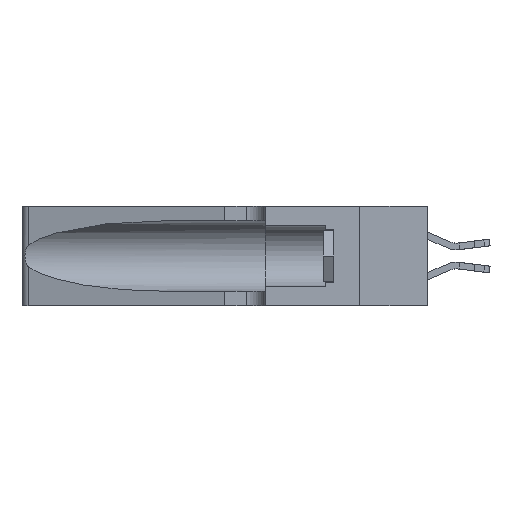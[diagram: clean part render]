
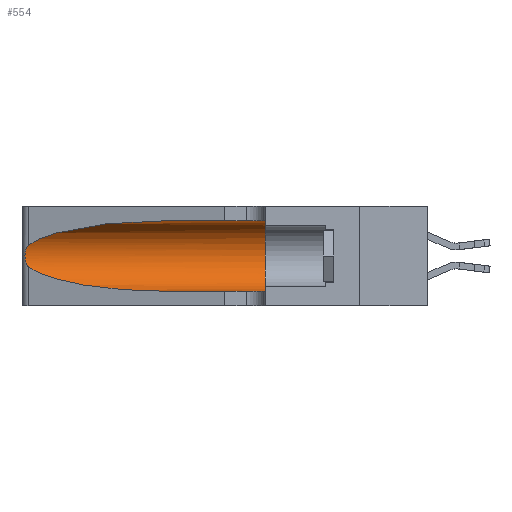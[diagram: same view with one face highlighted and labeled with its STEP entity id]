
A CAD part, left-side view. The second image highlights one B-rep face of the part: STEP entity #554.
In plain terms, the highlighted cylindrical face has radius 3.308 mm (diameter 6.617 mm), a partial arc.
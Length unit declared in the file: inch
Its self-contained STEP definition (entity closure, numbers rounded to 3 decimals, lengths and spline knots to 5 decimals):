
#235 = EDGE_LOOP ( 'NONE', ( #2622, #8775, #7417, #21664, #17510, #15327 ) ) ;
#342 = CARTESIAN_POINT ( 'NONE',  ( 0.25856, 1.23593, 0.16098 ) ) ;
#429 = CARTESIAN_POINT ( 'NONE',  ( 0.25487, 1.22718, 0.22369 ) ) ;
#525 = B_SPLINE_CURVE_WITH_KNOTS ( 'NONE', 3,
 ( #1756, #5209, #17364, #6971, #19101, #1903, #7247, #3805, #8969, #342, #2127, #16356, #9271, #3881 ),
 .UNSPECIFIED., .F., .F.,
 ( 4, 2, 2, 2, 2, 2, 4 ),
 ( 0., 0.00027, 0.00053, 0.00107, 0.0016, 0.00187, 0.00214 ),
 .UNSPECIFIED. ) ;
#554 = ADVANCED_FACE ( 'NONE', ( #5903 ), #7026, .F. ) ;
#969 = AXIS2_PLACEMENT_3D ( 'NONE', #9928, #2875, #3022 ) ;
#993 = VECTOR ( 'NONE', #12629, 39.37008 ) ;
#1394 = EDGE_CURVE ( 'NONE', #18174, #13818, #16700, .T. ) ;
#1395 = VERTEX_POINT ( 'NONE', #17748 ) ;
#1473 = CARTESIAN_POINT ( 'NONE',  ( 0.1305, 0.35, 0.05475 ) ) ;
#1756 = CARTESIAN_POINT ( 'NONE',  ( 0.25487, 1.22718, 0.22369 ) ) ;
#1782 = CARTESIAN_POINT ( 'NONE',  ( 0.25487, 1.22718, 0.14631 ) ) ;
#1903 = CARTESIAN_POINT ( 'NONE',  ( 0.26018, 1.23835, 0.19895 ) ) ;
#2127 = CARTESIAN_POINT ( 'NONE',  ( 0.25789, 1.23486, 0.15765 ) ) ;
#2622 = ORIENTED_EDGE ( 'NONE', *, *, #1394, .T. ) ;
#2875 = DIRECTION ( 'NONE',  ( 0., 1., 0. ) ) ;
#2895 = VERTEX_POINT ( 'NONE', #19126 ) ;
#2915 =( BOUNDED_CURVE ( )  B_SPLINE_CURVE ( 3, ( #1782, #10401, #10469, #22448 ),
 .UNSPECIFIED., .F., .F. ) 
 B_SPLINE_CURVE_WITH_KNOTS ( ( 4, 4 ),
 ( 3.44316, 4.71239 ),
 .UNSPECIFIED. ) 
 CURVE ( )  GEOMETRIC_REPRESENTATION_ITEM ( )  RATIONAL_B_SPLINE_CURVE ( ( 1., 0.87, 0.87, 1. ) ) 
 REPRESENTATION_ITEM ( '' )  );
#3022 = DIRECTION ( 'NONE',  ( 0., 0., 1. ) ) ;
#3223 = DIRECTION ( 'NONE',  ( 0., 0., -1. ) ) ;
#3502 = DIRECTION ( 'NONE',  ( 0., -1., 0. ) ) ;
#3805 = CARTESIAN_POINT ( 'NONE',  ( 0.26075, 1.23896, 0.178 ) ) ;
#3881 = CARTESIAN_POINT ( 'NONE',  ( 0.25487, 1.22718, 0.14631 ) ) ;
#3979 = CARTESIAN_POINT ( 'NONE',  ( 0.2373, 1.15595, 0.28018 ) ) ;
#5209 = CARTESIAN_POINT ( 'NONE',  ( 0.25555, 1.22994, 0.2215 ) ) ;
#5401 = LINE ( 'NONE', #12109, #21978 ) ;
#5612 = LINE ( 'NONE', #14020, #993 ) ;
#5903 = FACE_OUTER_BOUND ( 'NONE', #235, .T. ) ;
#6422 = CARTESIAN_POINT ( 'NONE',  ( 0.25487, 1.22718, 0.22369 ) ) ;
#6939 = CARTESIAN_POINT ( 'NONE',  ( 0.1305, 1.61858, 0.185 ) ) ;
#6971 = CARTESIAN_POINT ( 'NONE',  ( 0.25787, 1.23484, 0.2124 ) ) ;
#7026 = CYLINDRICAL_SURFACE ( 'NONE', #12128, 0.13025 ) ;
#7247 = CARTESIAN_POINT ( 'NONE',  ( 0.26075, 1.23896, 0.19203 ) ) ;
#7417 = ORIENTED_EDGE ( 'NONE', *, *, #16127, .T. ) ;
#8775 = ORIENTED_EDGE ( 'NONE', *, *, #13025, .T. ) ;
#8969 = CARTESIAN_POINT ( 'NONE',  ( 0.26017, 1.23833, 0.17102 ) ) ;
#9271 = CARTESIAN_POINT ( 'NONE',  ( 0.25555, 1.22993, 0.14849 ) ) ;
#9588 = VERTEX_POINT ( 'NONE', #15658 ) ;
#9928 = CARTESIAN_POINT ( 'NONE',  ( 0.1305, 0.35, 0.185 ) ) ;
#10401 = CARTESIAN_POINT ( 'NONE',  ( 0.2373, 1.15595, 0.08982 ) ) ;
#10469 = CARTESIAN_POINT ( 'NONE',  ( 0.18966, 0.96281, 0.05475 ) ) ;
#10640 = CIRCLE ( 'NONE', #969, 0.13025 ) ;
#10826 = CARTESIAN_POINT ( 'NONE',  ( 0.18966, 0.96281, 0.31525 ) ) ;
#12028 = VERTEX_POINT ( 'NONE', #1473 ) ;
#12109 = CARTESIAN_POINT ( 'NONE',  ( 0.1305, 1.61858, 0.05475 ) ) ;
#12128 = AXIS2_PLACEMENT_3D ( 'NONE', #6939, #3502, #3223 ) ;
#12629 = DIRECTION ( 'NONE',  ( 0., -1., 0. ) ) ;
#12920 = EDGE_CURVE ( 'NONE', #1395, #12028, #10640, .T. ) ;
#13025 = EDGE_CURVE ( 'NONE', #13818, #2895, #525, .T. ) ;
#13818 = VERTEX_POINT ( 'NONE', #6422 ) ;
#14020 = CARTESIAN_POINT ( 'NONE',  ( 0.1305, 1.61858, 0.31525 ) ) ;
#14285 = EDGE_CURVE ( 'NONE', #9588, #12028, #5401, .T. ) ;
#15327 = ORIENTED_EDGE ( 'NONE', *, *, #21451, .F. ) ;
#15658 = CARTESIAN_POINT ( 'NONE',  ( 0.1305, 0.72297, 0.05475 ) ) ;
#16127 = EDGE_CURVE ( 'NONE', #2895, #9588, #2915, .T. ) ;
#16356 = CARTESIAN_POINT ( 'NONE',  ( 0.25639, 1.23186, 0.15144 ) ) ;
#16700 =( BOUNDED_CURVE ( )  B_SPLINE_CURVE ( 3, ( #21074, #10826, #3979, #429 ),
 .UNSPECIFIED., .F., .T. ) 
 B_SPLINE_CURVE_WITH_KNOTS ( ( 4, 4 ),
 ( 1.5708, 2.84003 ),
 .UNSPECIFIED. ) 
 CURVE ( )  GEOMETRIC_REPRESENTATION_ITEM ( )  RATIONAL_B_SPLINE_CURVE ( ( 1., 0.87, 0.87, 1. ) ) 
 REPRESENTATION_ITEM ( '' )  );
#17364 = CARTESIAN_POINT ( 'NONE',  ( 0.25639, 1.23184, 0.21858 ) ) ;
#17510 = ORIENTED_EDGE ( 'NONE', *, *, #12920, .F. ) ;
#17748 = CARTESIAN_POINT ( 'NONE',  ( 0.1305, 0.35, 0.31525 ) ) ;
#17930 = CARTESIAN_POINT ( 'NONE',  ( 0.1305, 0.72297, 0.31525 ) ) ;
#18174 = VERTEX_POINT ( 'NONE', #17930 ) ;
#19031 = DIRECTION ( 'NONE',  ( 0., -1., 0. ) ) ;
#19101 = CARTESIAN_POINT ( 'NONE',  ( 0.25854, 1.2359, 0.20912 ) ) ;
#19126 = CARTESIAN_POINT ( 'NONE',  ( 0.25487, 1.22718, 0.14631 ) ) ;
#21074 = CARTESIAN_POINT ( 'NONE',  ( 0.1305, 0.72297, 0.31525 ) ) ;
#21451 = EDGE_CURVE ( 'NONE', #18174, #1395, #5612, .T. ) ;
#21664 = ORIENTED_EDGE ( 'NONE', *, *, #14285, .T. ) ;
#21978 = VECTOR ( 'NONE', #19031, 39.37008 ) ;
#22448 = CARTESIAN_POINT ( 'NONE',  ( 0.1305, 0.72297, 0.05475 ) ) ;
